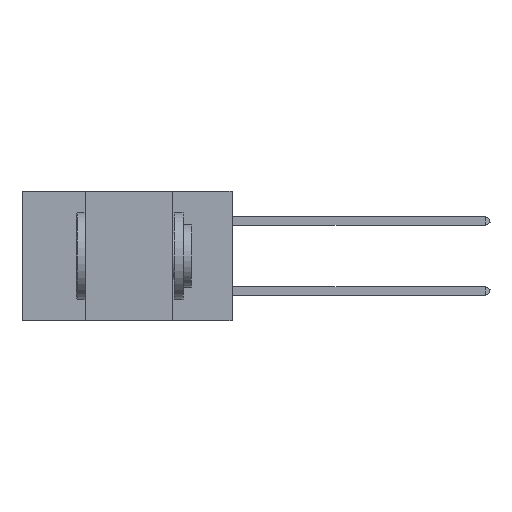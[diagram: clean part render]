
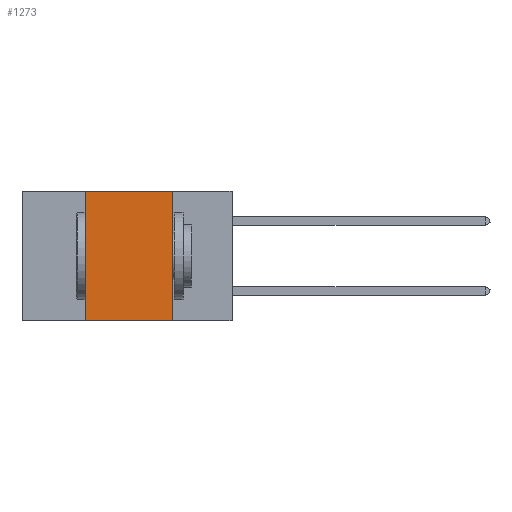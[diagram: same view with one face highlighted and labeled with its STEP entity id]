
A CAD part, left-side view. The second image highlights one B-rep face of the part: STEP entity #1273.
In plain terms, the highlighted planar face has unit normal (-1, 0, 0).
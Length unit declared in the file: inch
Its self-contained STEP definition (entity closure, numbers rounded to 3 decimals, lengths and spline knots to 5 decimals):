
#414 = VERTEX_POINT ( 'NONE', #1783 ) ;
#766 = EDGE_CURVE ( 'NONE', #6253, #414, #9651, .T. ) ;
#1024 = EDGE_CURVE ( 'NONE', #414, #5095, #12884, .T. ) ;
#1273 = ADVANCED_FACE ( 'NONE', ( #13868 ), #6209, .F. ) ;
#1783 = CARTESIAN_POINT ( 'NONE',  ( 0., 0.17, 0. ) ) ;
#1903 = CARTESIAN_POINT ( 'NONE',  ( 0., 0.17, -0.37 ) ) ;
#2992 = ORIENTED_EDGE ( 'NONE', *, *, #5037, .F. ) ;
#3070 = CARTESIAN_POINT ( 'NONE',  ( 0., 0.42, 0. ) ) ;
#3515 = EDGE_CURVE ( 'NONE', #11018, #5095, #14642, .T. ) ;
#3678 = VECTOR ( 'NONE', #12705, 39.37008 ) ;
#3691 = DIRECTION ( 'NONE',  ( 1., 0., 0. ) ) ;
#4338 = DIRECTION ( 'NONE',  ( 0., 0., -1. ) ) ;
#4374 = VECTOR ( 'NONE', #8834, 39.37008 ) ;
#4925 = CARTESIAN_POINT ( 'NONE',  ( 0., 0.6, 0. ) ) ;
#5037 = EDGE_CURVE ( 'NONE', #11018, #6253, #9856, .T. ) ;
#5095 = VERTEX_POINT ( 'NONE', #1903 ) ;
#5664 = ORIENTED_EDGE ( 'NONE', *, *, #766, .F. ) ;
#6024 = ORIENTED_EDGE ( 'NONE', *, *, #3515, .T. ) ;
#6209 = PLANE ( 'NONE',  #6946 ) ;
#6253 = VERTEX_POINT ( 'NONE', #14569 ) ;
#6902 = VECTOR ( 'NONE', #13107, 39.37008 ) ;
#6946 = AXIS2_PLACEMENT_3D ( 'NONE', #4925, #3691, #4338 ) ;
#8301 = ORIENTED_EDGE ( 'NONE', *, *, #1024, .F. ) ;
#8339 = CARTESIAN_POINT ( 'NONE',  ( 0., 0.42, -0.37 ) ) ;
#8719 = CARTESIAN_POINT ( 'NONE',  ( 0., 0.6, 0. ) ) ;
#8834 = DIRECTION ( 'NONE',  ( 0., 0., -1. ) ) ;
#9651 = LINE ( 'NONE', #8719, #3678 ) ;
#9856 = LINE ( 'NONE', #3070, #6902 ) ;
#10429 = CARTESIAN_POINT ( 'NONE',  ( 0., 0.17, 0. ) ) ;
#11018 = VERTEX_POINT ( 'NONE', #8339 ) ;
#11188 = CARTESIAN_POINT ( 'NONE',  ( 0., 0.6, -0.37 ) ) ;
#11772 = VECTOR ( 'NONE', #13371, 39.37008 ) ;
#11835 = EDGE_LOOP ( 'NONE', ( #8301, #5664, #2992, #6024 ) ) ;
#12705 = DIRECTION ( 'NONE',  ( 0., -1., 0. ) ) ;
#12884 = LINE ( 'NONE', #10429, #4374 ) ;
#13107 = DIRECTION ( 'NONE',  ( 0., 0., 1. ) ) ;
#13371 = DIRECTION ( 'NONE',  ( 0., -1., 0. ) ) ;
#13868 = FACE_OUTER_BOUND ( 'NONE', #11835, .T. ) ;
#14569 = CARTESIAN_POINT ( 'NONE',  ( 0., 0.42, 0. ) ) ;
#14642 = LINE ( 'NONE', #11188, #11772 ) ;
